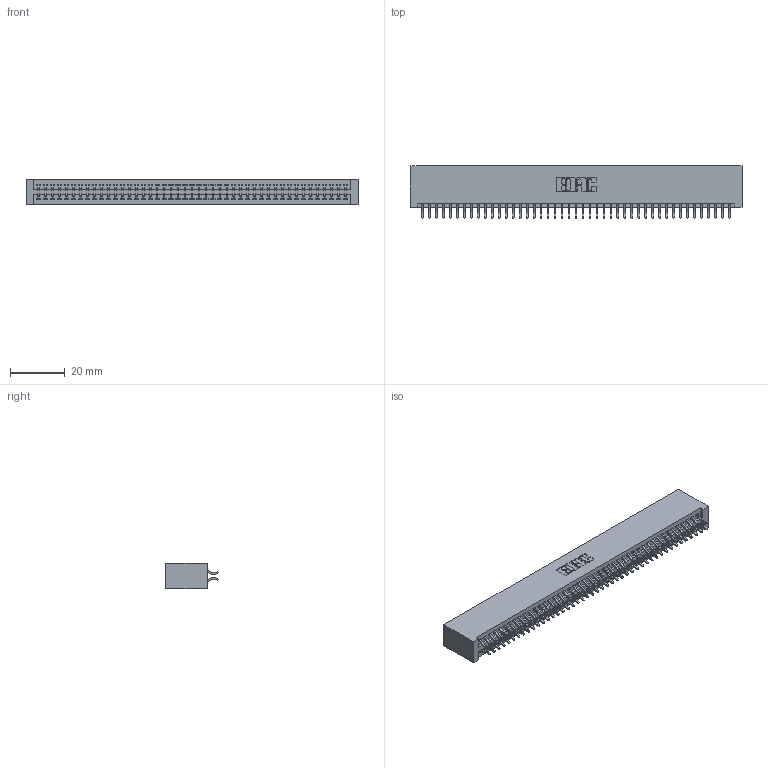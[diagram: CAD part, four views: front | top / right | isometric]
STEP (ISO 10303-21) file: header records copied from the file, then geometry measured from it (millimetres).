
FILE_DESCRIPTION (( 'STEP AP203' ), '1' );
FILE_NAME ('345-090-556-201.STEP', '2019-11-01T16:51:21', ( '' ), ( '' ), 'SwSTEP 2.0', 'SolidWorks 2016', '' );
FILE_SCHEMA (( 'CONFIG_CONTROL_DESIGN' ));
Length unit declared in the file: inch
Products named in the file (3): 345 Part_No Mounting Lugs; 345-090-556-201; 345-292-001_556 Tail
Assembly tree (91 placements, depth 2):
  345-090-556-201
    345 Part_No Mounting Lugs
    345-292-001_556 Tail  x90
Bounding box: 120.9 x 19.24 x 9.4 mm (x, y, z)
Volume: 12384.9 mm3; surface area: 18589.6 mm2
Topology: 91 solids, 91 shells, 5158 faces, 15347 edges, 10110 vertices
Faces by surface type: plane 3406, cylinder 1752
Entity records: 34847 total; most frequent: CARTESIAN_POINT 5852, ORIENTED_EDGE 5774, DIRECTION 5139, EDGE_CURVE 2887, VECTOR 2575, LINE 2575, VERTEX_POINT 1922, AXIS2_PLACEMENT_3D 1282
